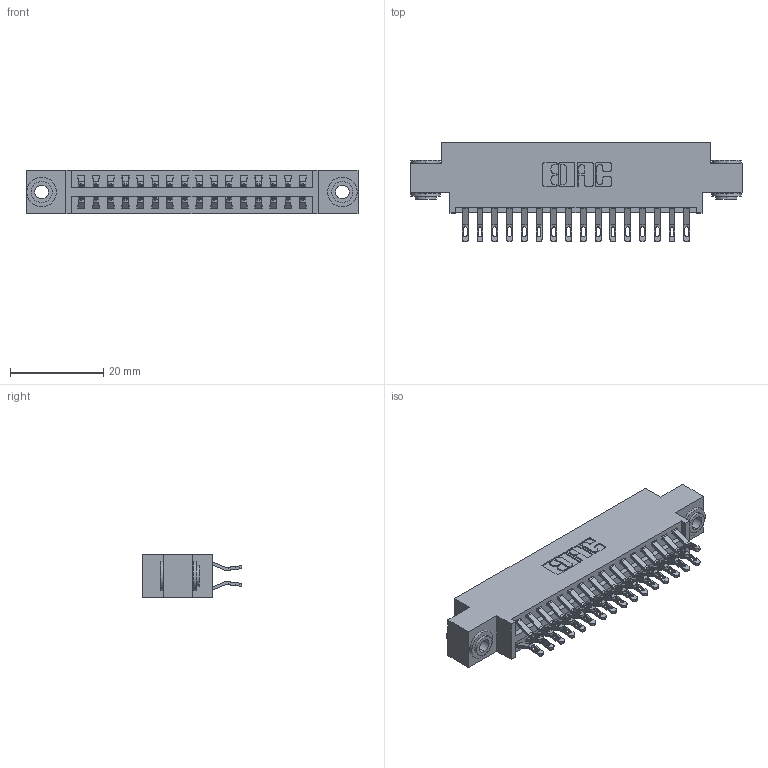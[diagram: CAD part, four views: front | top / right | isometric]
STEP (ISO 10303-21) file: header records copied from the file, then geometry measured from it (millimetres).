
FILE_DESCRIPTION (( 'STEP AP203' ), '1' );
FILE_NAME ('396-032-555-803.STEP', '2019-11-01T20:06:55', ( '' ), ( '' ), 'SwSTEP 2.0', 'SolidWorks 2016', '' );
FILE_SCHEMA (( 'CONFIG_CONTROL_DESIGN' ));
Length unit declared in the file: inch
Products named in the file (4): 346 Part_0.170 Offset - 0.156 Dia-TH; 345-292-001_555 Tail; 345-250-002_345-250-002-102; 396-032-555-803
Assembly tree (35 placements, depth 2):
  396-032-555-803
    346 Part_0.170 Offset - 0.156 Dia-TH
    345-292-001_555 Tail  x32
    345-250-002_345-250-002-102  x2
Bounding box: 71.37 x 21.46 x 9.4 mm (x, y, z)
Volume: 6715.5 mm3; surface area: 9546.9 mm2
Topology: 35 solids, 35 shells, 2020 faces, 6273 edges, 4178 vertices
Faces by surface type: plane 1146, cylinder 866, cone 8
Entity records: 15050 total; most frequent: CARTESIAN_POINT 2529, ORIENTED_EDGE 2426, DIRECTION 2279, EDGE_CURVE 1213, VECTOR 973, LINE 973, VERTEX_POINT 806, AXIS2_PLACEMENT_3D 653
